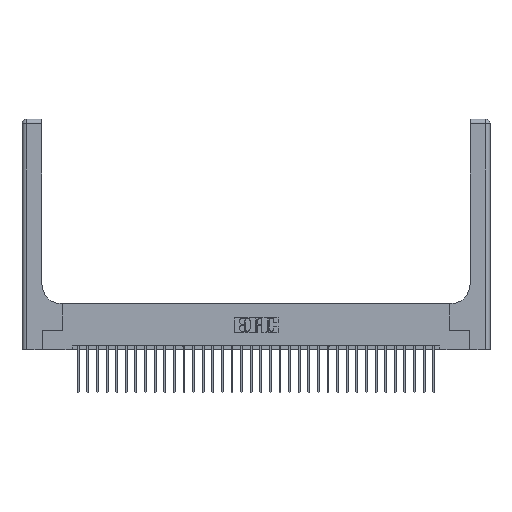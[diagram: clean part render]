
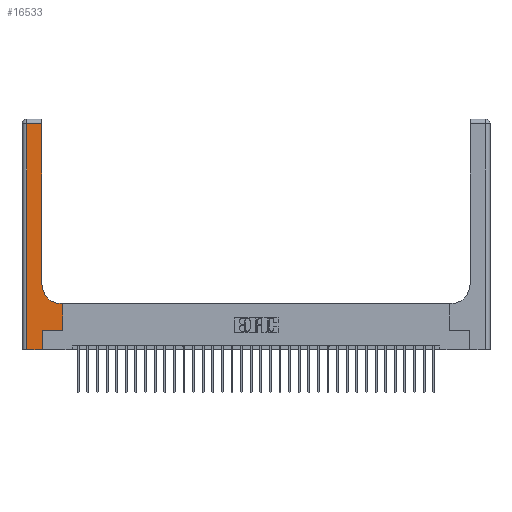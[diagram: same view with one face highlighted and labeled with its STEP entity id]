
A CAD part, top view. The second image highlights one B-rep face of the part: STEP entity #16533.
In plain terms, the highlighted planar face has unit normal (0, 0, 1).
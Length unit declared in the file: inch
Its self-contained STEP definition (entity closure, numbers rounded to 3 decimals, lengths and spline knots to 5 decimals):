
#543 = EDGE_CURVE ( 'NONE', #5457, #3422, #6860, .T. ) ;
#946 = DIRECTION ( 'NONE',  ( 0., 1., 0. ) ) ;
#1505 = EDGE_CURVE ( 'NONE', #14491, #10988, #2367, .T. ) ;
#1583 = DIRECTION ( 'NONE',  ( 0., 0., -1. ) ) ;
#1941 = CARTESIAN_POINT ( 'NONE',  ( 0.265, 0.25, 0.37 ) ) ;
#2367 = LINE ( 'NONE', #18279, #23053 ) ;
#2722 = FACE_OUTER_BOUND ( 'NONE', #8789, .T. ) ;
#2987 = CARTESIAN_POINT ( 'NONE',  ( 0.26, 3., 0.37 ) ) ;
#3302 = DIRECTION ( 'NONE',  ( 1., 0., 0. ) ) ;
#3422 = VERTEX_POINT ( 'NONE', #18806 ) ;
#4553 = CIRCLE ( 'NONE', #11177, 0.25 ) ;
#4865 = CARTESIAN_POINT ( 'NONE',  ( 0.528, 0.6, 0.37 ) ) ;
#5457 = VERTEX_POINT ( 'NONE', #29427 ) ;
#5609 = CARTESIAN_POINT ( 'NONE',  ( 0.528, 0.25, 0.37 ) ) ;
#6860 = LINE ( 'NONE', #8023, #24913 ) ;
#6868 = LINE ( 'NONE', #16045, #23813 ) ;
#7838 = VECTOR ( 'NONE', #25740, 39.37008 ) ;
#8023 = CARTESIAN_POINT ( 'NONE',  ( 0.265, 0., 0.37 ) ) ;
#8789 = EDGE_LOOP ( 'NONE', ( #13103, #14515, #12067, #22385, #23955, #13691, #17540, #28616, #24547 ) ) ;
#9087 = EDGE_CURVE ( 'NONE', #29593, #14509, #4553, .T. ) ;
#10009 = VECTOR ( 'NONE', #20631, 39.37008 ) ;
#10270 = CARTESIAN_POINT ( 'NONE',  ( 0.528, 0.25, 0.37 ) ) ;
#10988 = VERTEX_POINT ( 'NONE', #20068 ) ;
#11177 = AXIS2_PLACEMENT_3D ( 'NONE', #19642, #27055, #3302 ) ;
#11246 = EDGE_CURVE ( 'NONE', #14244, #14491, #17005, .T. ) ;
#11644 = EDGE_CURVE ( 'NONE', #3422, #25493, #19938, .T. ) ;
#12067 = ORIENTED_EDGE ( 'NONE', *, *, #1505, .T. ) ;
#12772 = EDGE_CURVE ( 'NONE', #25493, #25948, #13575, .T. ) ;
#13103 = ORIENTED_EDGE ( 'NONE', *, *, #16882, .T. ) ;
#13575 = LINE ( 'NONE', #10270, #22059 ) ;
#13691 = ORIENTED_EDGE ( 'NONE', *, *, #11644, .T. ) ;
#14244 = VERTEX_POINT ( 'NONE', #21097 ) ;
#14491 = VERTEX_POINT ( 'NONE', #21961 ) ;
#14509 = VERTEX_POINT ( 'NONE', #14950 ) ;
#14515 = ORIENTED_EDGE ( 'NONE', *, *, #11246, .T. ) ;
#14681 = DIRECTION ( 'NONE',  ( 0., 1., 0. ) ) ;
#14710 = DIRECTION ( 'NONE',  ( -1., 0., 0. ) ) ;
#14950 = CARTESIAN_POINT ( 'NONE',  ( 0.26, 0.85, 0.37 ) ) ;
#15518 = VECTOR ( 'NONE', #14710, 39.37008 ) ;
#15736 = CARTESIAN_POINT ( 'NONE',  ( 0., 3., 0.37 ) ) ;
#15843 = DIRECTION ( 'NONE',  ( 0., -1., 0. ) ) ;
#15922 = EDGE_CURVE ( 'NONE', #10988, #5457, #6868, .T. ) ;
#16045 = CARTESIAN_POINT ( 'NONE',  ( 0., 0., 0.37 ) ) ;
#16533 = ADVANCED_FACE ( 'NONE', ( #2722 ), #29866, .F. ) ;
#16882 = EDGE_CURVE ( 'NONE', #14509, #14244, #21887, .T. ) ;
#17005 = LINE ( 'NONE', #28080, #7838 ) ;
#17540 = ORIENTED_EDGE ( 'NONE', *, *, #12772, .T. ) ;
#18279 = CARTESIAN_POINT ( 'NONE',  ( 0.06, 3., 0.37 ) ) ;
#18396 = DIRECTION ( 'NONE',  ( 1., 0., 0. ) ) ;
#18806 = CARTESIAN_POINT ( 'NONE',  ( 0.265, 0.25, 0.37 ) ) ;
#19092 = EDGE_CURVE ( 'NONE', #25948, #29593, #20654, .T. ) ;
#19642 = CARTESIAN_POINT ( 'NONE',  ( 0.51, 0.85, 0.37 ) ) ;
#19938 = LINE ( 'NONE', #1941, #10009 ) ;
#20068 = CARTESIAN_POINT ( 'NONE',  ( 0.06, 0., 0.37 ) ) ;
#20461 = DIRECTION ( 'NONE',  ( -1., 0., 0. ) ) ;
#20631 = DIRECTION ( 'NONE',  ( 1., 0., 0. ) ) ;
#20654 = LINE ( 'NONE', #26467, #15518 ) ;
#21097 = CARTESIAN_POINT ( 'NONE',  ( 0.26, 2.94, 0.37 ) ) ;
#21887 = LINE ( 'NONE', #2987, #28555 ) ;
#21961 = CARTESIAN_POINT ( 'NONE',  ( 0.06, 2.94, 0.37 ) ) ;
#22059 = VECTOR ( 'NONE', #29202, 39.37008 ) ;
#22385 = ORIENTED_EDGE ( 'NONE', *, *, #15922, .T. ) ;
#23053 = VECTOR ( 'NONE', #15843, 39.37008 ) ;
#23813 = VECTOR ( 'NONE', #18396, 39.37008 ) ;
#23955 = ORIENTED_EDGE ( 'NONE', *, *, #543, .T. ) ;
#24547 = ORIENTED_EDGE ( 'NONE', *, *, #9087, .T. ) ;
#24913 = VECTOR ( 'NONE', #946, 39.37008 ) ;
#25493 = VERTEX_POINT ( 'NONE', #5609 ) ;
#25740 = DIRECTION ( 'NONE',  ( -1., 0., 0. ) ) ;
#25948 = VERTEX_POINT ( 'NONE', #4865 ) ;
#26154 = CARTESIAN_POINT ( 'NONE',  ( 0.51, 0.6, 0.37 ) ) ;
#26467 = CARTESIAN_POINT ( 'NONE',  ( 0.26, 0.6, 0.37 ) ) ;
#27055 = DIRECTION ( 'NONE',  ( 0., 0., -1. ) ) ;
#28080 = CARTESIAN_POINT ( 'NONE',  ( 0., 2.94, 0.37 ) ) ;
#28555 = VECTOR ( 'NONE', #14681, 39.37008 ) ;
#28616 = ORIENTED_EDGE ( 'NONE', *, *, #19092, .T. ) ;
#29202 = DIRECTION ( 'NONE',  ( 0., 1., 0. ) ) ;
#29427 = CARTESIAN_POINT ( 'NONE',  ( 0.265, 0., 0.37 ) ) ;
#29593 = VERTEX_POINT ( 'NONE', #26154 ) ;
#29864 = AXIS2_PLACEMENT_3D ( 'NONE', #15736, #1583, #20461 ) ;
#29866 = PLANE ( 'NONE',  #29864 ) ;
